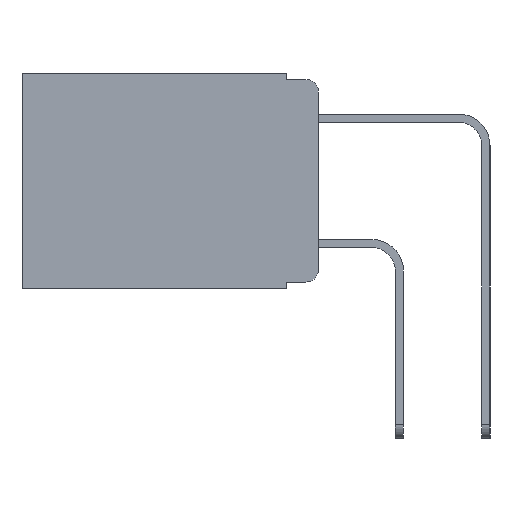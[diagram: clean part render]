
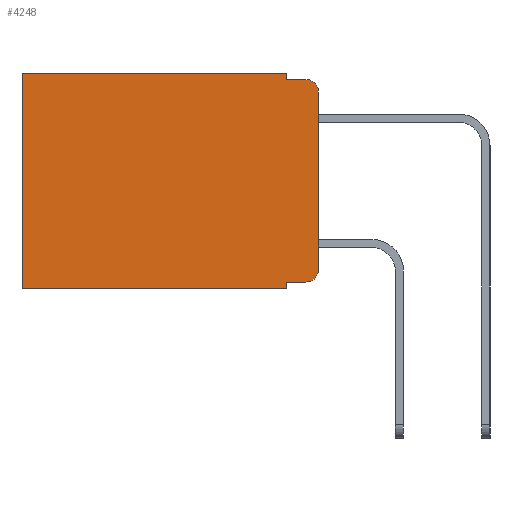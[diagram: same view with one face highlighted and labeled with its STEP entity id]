
A CAD part, left-side view. The second image highlights one B-rep face of the part: STEP entity #4248.
In plain terms, the highlighted planar face has unit normal (-1, 0, 0).
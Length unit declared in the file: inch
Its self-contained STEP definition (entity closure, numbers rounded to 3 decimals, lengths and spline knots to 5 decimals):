
#59 = EDGE_CURVE ( 'NONE', #112, #7741, #1784, .T. ) ;
#69 = ORIENTED_EDGE ( 'NONE', *, *, #10027, .F. ) ;
#112 = VERTEX_POINT ( 'NONE', #8366 ) ;
#204 = ORIENTED_EDGE ( 'NONE', *, *, #6985, .F. ) ;
#859 = ORIENTED_EDGE ( 'NONE', *, *, #11668, .F. ) ;
#964 = EDGE_CURVE ( 'NONE', #112, #9909, #7899, .T. ) ;
#1162 = FACE_OUTER_BOUND ( 'NONE', #1392, .T. ) ;
#1280 = DIRECTION ( 'NONE',  ( 0., 1., 0. ) ) ;
#1392 = EDGE_LOOP ( 'NONE', ( #2229, #1685, #4043, #859, #10278, #1449, #69, #204, #5733, #5341 ) ) ;
#1449 = ORIENTED_EDGE ( 'NONE', *, *, #11418, .T. ) ;
#1655 = AXIS2_PLACEMENT_3D ( 'NONE', #4717, #12015, #6596 ) ;
#1685 = ORIENTED_EDGE ( 'NONE', *, *, #964, .T. ) ;
#1784 = LINE ( 'NONE', #10772, #11633 ) ;
#2229 = ORIENTED_EDGE ( 'NONE', *, *, #59, .F. ) ;
#2298 = DIRECTION ( 'NONE',  ( -1., 0., 0. ) ) ;
#2302 = CARTESIAN_POINT ( 'NONE',  ( 0.298, 0., -0.343 ) ) ;
#2414 = CARTESIAN_POINT ( 'NONE',  ( 0.298, 0.051, -0.01 ) ) ;
#2446 = VERTEX_POINT ( 'NONE', #7590 ) ;
#2804 = CARTESIAN_POINT ( 'NONE',  ( 0.298, 0.051, -0.333 ) ) ;
#3148 = AXIS2_PLACEMENT_3D ( 'NONE', #9892, #4703, #4695 ) ;
#3603 = LINE ( 'NONE', #10125, #7907 ) ;
#3734 = DIRECTION ( 'NONE',  ( 0., 0., -1. ) ) ;
#3952 = CARTESIAN_POINT ( 'NONE',  ( 0.298, 0.051, 0. ) ) ;
#3961 = VERTEX_POINT ( 'NONE', #5258 ) ;
#4043 = ORIENTED_EDGE ( 'NONE', *, *, #5932, .F. ) ;
#4248 = ADVANCED_FACE ( 'NONE', ( #1162 ), #10258, .F. ) ;
#4285 = CARTESIAN_POINT ( 'NONE',  ( 0.298, 0.473, 0. ) ) ;
#4288 = VECTOR ( 'NONE', #11965, 39.37008 ) ;
#4695 = DIRECTION ( 'NONE',  ( 0., 0., -1. ) ) ;
#4703 = DIRECTION ( 'NONE',  ( -1., 0., 0. ) ) ;
#4717 = CARTESIAN_POINT ( 'NONE',  ( 0.298, 0., 0. ) ) ;
#4817 = EDGE_CURVE ( 'NONE', #5860, #3961, #6441, .T. ) ;
#5258 = CARTESIAN_POINT ( 'NONE',  ( 0.298, 0.02, -0.333 ) ) ;
#5270 = LINE ( 'NONE', #7365, #7684 ) ;
#5341 = ORIENTED_EDGE ( 'NONE', *, *, #5732, .T. ) ;
#5556 = VERTEX_POINT ( 'NONE', #3952 ) ;
#5576 = DIRECTION ( 'NONE',  ( 0., -1., 0. ) ) ;
#5732 = EDGE_CURVE ( 'NONE', #3961, #7741, #9726, .T. ) ;
#5733 = ORIENTED_EDGE ( 'NONE', *, *, #4817, .T. ) ;
#5787 = VERTEX_POINT ( 'NONE', #4285 ) ;
#5860 = VERTEX_POINT ( 'NONE', #11682 ) ;
#5932 = EDGE_CURVE ( 'NONE', #6966, #9909, #5270, .T. ) ;
#5986 = AXIS2_PLACEMENT_3D ( 'NONE', #7872, #2298, #8845 ) ;
#6441 = LINE ( 'NONE', #2804, #4288 ) ;
#6596 = DIRECTION ( 'NONE',  ( 0., 0., -1. ) ) ;
#6966 = VERTEX_POINT ( 'NONE', #2414 ) ;
#6985 = EDGE_CURVE ( 'NONE', #5860, #9968, #11394, .T. ) ;
#7094 = VECTOR ( 'NONE', #10769, 39.37008 ) ;
#7154 = VECTOR ( 'NONE', #1280, 39.37008 ) ;
#7324 = EDGE_CURVE ( 'NONE', #5556, #5787, #7652, .T. ) ;
#7365 = CARTESIAN_POINT ( 'NONE',  ( 0.298, 0.051, -0.01 ) ) ;
#7371 = VECTOR ( 'NONE', #7603, 39.37008 ) ;
#7590 = CARTESIAN_POINT ( 'NONE',  ( 0.298, 0.473, -0.343 ) ) ;
#7603 = DIRECTION ( 'NONE',  ( 0., 1., 0. ) ) ;
#7652 = LINE ( 'NONE', #12098, #7371 ) ;
#7684 = VECTOR ( 'NONE', #5576, 39.37008 ) ;
#7741 = VERTEX_POINT ( 'NONE', #8257 ) ;
#7872 = CARTESIAN_POINT ( 'NONE',  ( 0.298, 0.02, -0.313 ) ) ;
#7899 = CIRCLE ( 'NONE', #3148, 0.02 ) ;
#7907 = VECTOR ( 'NONE', #11034, 39.37008 ) ;
#8257 = CARTESIAN_POINT ( 'NONE',  ( 0.298, 0., -0.313 ) ) ;
#8366 = CARTESIAN_POINT ( 'NONE',  ( 0.298, 0., -0.03 ) ) ;
#8681 = CARTESIAN_POINT ( 'NONE',  ( 0.298, 0.02, -0.01 ) ) ;
#8845 = DIRECTION ( 'NONE',  ( 0., 0., -1. ) ) ;
#9278 = CARTESIAN_POINT ( 'NONE',  ( 0.298, 0.051, 0. ) ) ;
#9616 = LINE ( 'NONE', #2302, #7154 ) ;
#9726 = CIRCLE ( 'NONE', #5986, 0.02 ) ;
#9844 = CARTESIAN_POINT ( 'NONE',  ( 0.298, 0.051, 0. ) ) ;
#9892 = CARTESIAN_POINT ( 'NONE',  ( 0.298, 0.02, -0.03 ) ) ;
#9909 = VERTEX_POINT ( 'NONE', #8681 ) ;
#9934 = VECTOR ( 'NONE', #3734, 39.37008 ) ;
#9968 = VERTEX_POINT ( 'NONE', #10548 ) ;
#10027 = EDGE_CURVE ( 'NONE', #9968, #2446, #9616, .T. ) ;
#10125 = CARTESIAN_POINT ( 'NONE',  ( 0.298, 0.473, 0. ) ) ;
#10258 = PLANE ( 'NONE',  #1655 ) ;
#10278 = ORIENTED_EDGE ( 'NONE', *, *, #7324, .T. ) ;
#10548 = CARTESIAN_POINT ( 'NONE',  ( 0.298, 0.051, -0.343 ) ) ;
#10769 = DIRECTION ( 'NONE',  ( 0., 0., -1. ) ) ;
#10772 = CARTESIAN_POINT ( 'NONE',  ( 0.298, 0., 0. ) ) ;
#10788 = DIRECTION ( 'NONE',  ( 0., 0., -1. ) ) ;
#11034 = DIRECTION ( 'NONE',  ( 0., 0., -1. ) ) ;
#11394 = LINE ( 'NONE', #9844, #7094 ) ;
#11418 = EDGE_CURVE ( 'NONE', #5787, #2446, #3603, .T. ) ;
#11633 = VECTOR ( 'NONE', #10788, 39.37008 ) ;
#11668 = EDGE_CURVE ( 'NONE', #5556, #6966, #11731, .T. ) ;
#11682 = CARTESIAN_POINT ( 'NONE',  ( 0.298, 0.051, -0.333 ) ) ;
#11731 = LINE ( 'NONE', #9278, #9934 ) ;
#11965 = DIRECTION ( 'NONE',  ( 0., -1., 0. ) ) ;
#12015 = DIRECTION ( 'NONE',  ( 1., 0., 0. ) ) ;
#12098 = CARTESIAN_POINT ( 'NONE',  ( 0.298, 0., 0. ) ) ;
